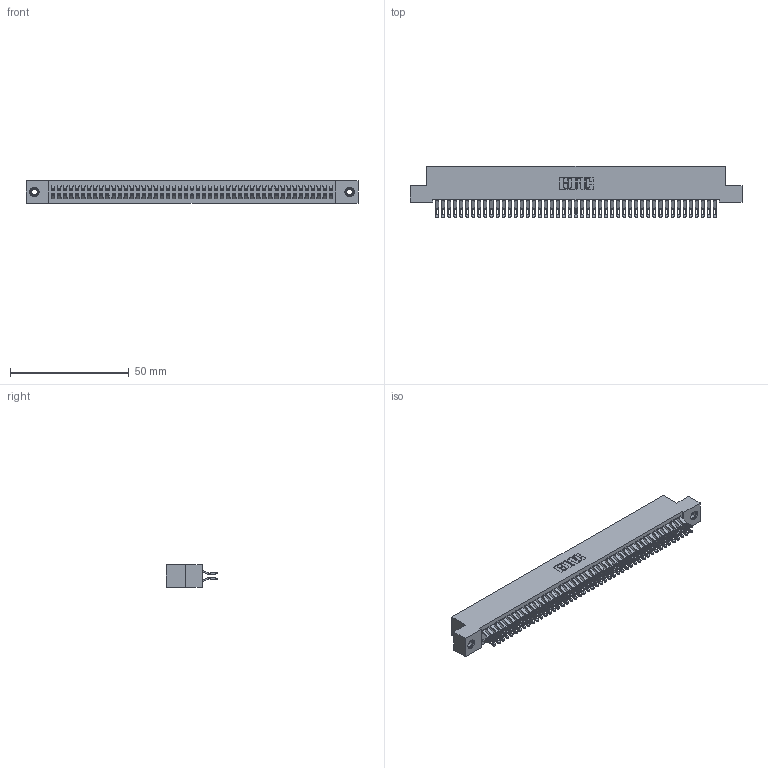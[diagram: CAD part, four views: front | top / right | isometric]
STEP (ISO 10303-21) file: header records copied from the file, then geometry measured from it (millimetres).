
FILE_DESCRIPTION (( 'STEP AP203' ), '1' );
FILE_NAME ('392-094-555-207.STEP', '2018-08-18T09:10:06', ( '' ), ( '' ), 'SwSTEP 2.0', 'SolidWorks 2016', '' );
FILE_SCHEMA (( 'CONFIG_CONTROL_DESIGN' ));
Length unit declared in the file: inch
Products named in the file (4): 392-094-555-207; 342 Part_TI; 345-292-001_555 Tail; 345-250-001_345-250-005-103
Assembly tree (97 placements, depth 2):
  392-094-555-207
    342 Part_TI
    345-292-001_555 Tail  x94
    345-250-001_345-250-005-103  x2
Bounding box: 139.7 x 21.47 x 9.4 mm (x, y, z)
Volume: 12824.2 mm3; surface area: 21933.1 mm2
Topology: 97 solids, 97 shells, 5622 faces, 17637 edges, 11750 vertices
Faces by surface type: plane 3294, cylinder 2312, cone 12, torus 4
Entity records: 30970 total; most frequent: CARTESIAN_POINT 5143, ORIENTED_EDGE 5042, DIRECTION 4387, EDGE_CURVE 2521, LINE 2353, VECTOR 2353, VERTEX_POINT 1676, AXIS2_PLACEMENT_3D 1017
